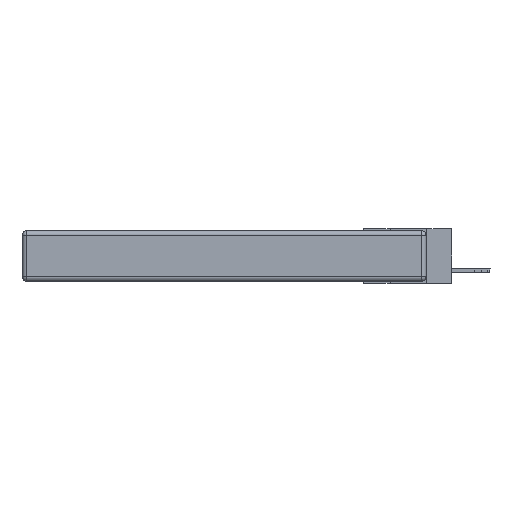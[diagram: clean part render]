
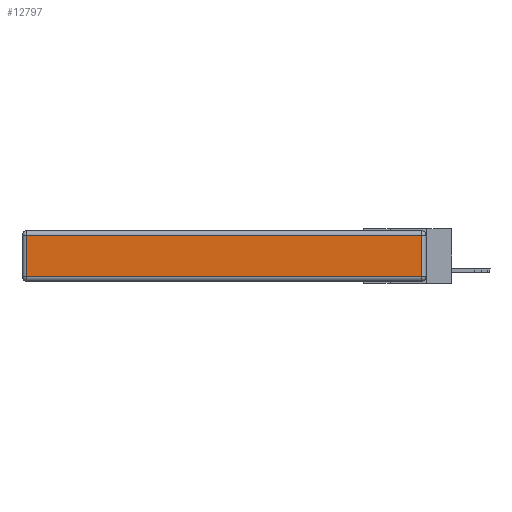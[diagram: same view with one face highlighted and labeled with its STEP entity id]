
A CAD part, left-side view. The second image highlights one B-rep face of the part: STEP entity #12797.
In plain terms, the highlighted planar face has unit normal (-1, 0, 0).
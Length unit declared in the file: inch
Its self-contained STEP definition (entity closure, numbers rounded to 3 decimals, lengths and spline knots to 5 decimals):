
#247 = CARTESIAN_POINT ( 'NONE',  ( 0., 2.75, -0.03 ) ) ;
#752 = CARTESIAN_POINT ( 'NONE',  ( 0., 0.03, -0.343 ) ) ;
#859 = CARTESIAN_POINT ( 'NONE',  ( 0., 2.72, -0.343 ) ) ;
#945 = ORIENTED_EDGE ( 'NONE', *, *, #13792, .T. ) ;
#1222 = PLANE ( 'NONE',  #20373 ) ;
#1736 = VERTEX_POINT ( 'NONE', #19584 ) ;
#1989 = DIRECTION ( 'NONE',  ( 0., 1., 0. ) ) ;
#2705 = ORIENTED_EDGE ( 'NONE', *, *, #18554, .T. ) ;
#2982 = DIRECTION ( 'NONE',  ( -1., 0., 0. ) ) ;
#3133 = CARTESIAN_POINT ( 'NONE',  ( 0., 0., -0.343 ) ) ;
#3323 = LINE ( 'NONE', #859, #20688 ) ;
#3549 = ORIENTED_EDGE ( 'NONE', *, *, #5910, .T. ) ;
#5096 = ORIENTED_EDGE ( 'NONE', *, *, #8262, .T. ) ;
#5546 = VECTOR ( 'NONE', #19931, 39.37008 ) ;
#5910 = EDGE_CURVE ( 'NONE', #1736, #12259, #9579, .T. ) ;
#6100 = CARTESIAN_POINT ( 'NONE',  ( 0., 0.03, -0.313 ) ) ;
#7533 = FACE_OUTER_BOUND ( 'NONE', #14655, .T. ) ;
#8171 = DIRECTION ( 'NONE',  ( 0., 0., 1. ) ) ;
#8262 = EDGE_CURVE ( 'NONE', #12259, #9504, #9220, .T. ) ;
#8766 = VECTOR ( 'NONE', #10166, 39.37008 ) ;
#9220 = LINE ( 'NONE', #752, #5546 ) ;
#9504 = VERTEX_POINT ( 'NONE', #12260 ) ;
#9579 = LINE ( 'NONE', #20165, #8766 ) ;
#10166 = DIRECTION ( 'NONE',  ( 0., -1., 0. ) ) ;
#11467 = VECTOR ( 'NONE', #1989, 39.37008 ) ;
#12259 = VERTEX_POINT ( 'NONE', #6100 ) ;
#12260 = CARTESIAN_POINT ( 'NONE',  ( 0., 0.03, -0.03 ) ) ;
#12797 = ADVANCED_FACE ( 'NONE', ( #7533 ), #1222, .T. ) ;
#13280 = LINE ( 'NONE', #247, #11467 ) ;
#13637 = VERTEX_POINT ( 'NONE', #20172 ) ;
#13792 = EDGE_CURVE ( 'NONE', #9504, #13637, #13280, .T. ) ;
#14655 = EDGE_LOOP ( 'NONE', ( #3549, #5096, #945, #2705 ) ) ;
#15962 = DIRECTION ( 'NONE',  ( 0., 0., -1. ) ) ;
#18554 = EDGE_CURVE ( 'NONE', #13637, #1736, #3323, .T. ) ;
#19584 = CARTESIAN_POINT ( 'NONE',  ( 0., 2.72, -0.313 ) ) ;
#19931 = DIRECTION ( 'NONE',  ( 0., 0., 1. ) ) ;
#20165 = CARTESIAN_POINT ( 'NONE',  ( 0., 0., -0.313 ) ) ;
#20172 = CARTESIAN_POINT ( 'NONE',  ( 0., 2.72, -0.03 ) ) ;
#20373 = AXIS2_PLACEMENT_3D ( 'NONE', #3133, #2982, #8171 ) ;
#20688 = VECTOR ( 'NONE', #15962, 39.37008 ) ;
